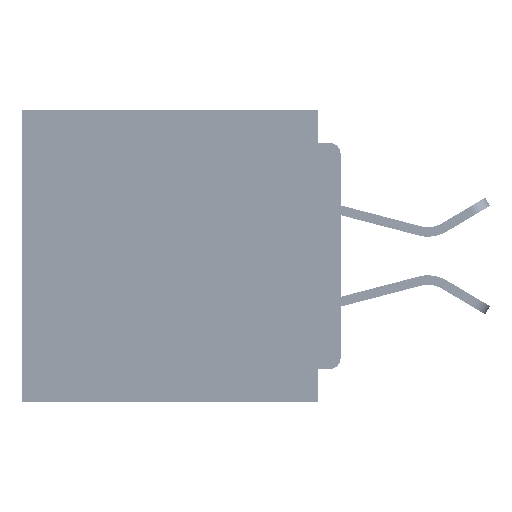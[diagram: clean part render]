
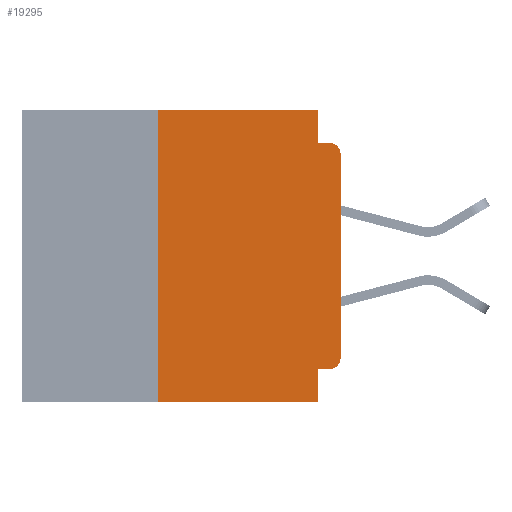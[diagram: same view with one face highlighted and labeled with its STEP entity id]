
A CAD part, left-side view. The second image highlights one B-rep face of the part: STEP entity #19295.
In plain terms, the highlighted planar face has unit normal (-1, 0, 0).
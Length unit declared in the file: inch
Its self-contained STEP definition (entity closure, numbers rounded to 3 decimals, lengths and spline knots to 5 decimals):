
#38 = PLANE ( 'NONE',  #16601 ) ;
#357 = CARTESIAN_POINT ( 'NONE',  ( 0., 0.25, -0.4 ) ) ;
#648 = DIRECTION ( 'NONE',  ( 0., 0., -1. ) ) ;
#830 = LINE ( 'NONE', #15773, #28668 ) ;
#1079 = VECTOR ( 'NONE', #26083, 39.37008 ) ;
#1973 = VERTEX_POINT ( 'NONE', #3109 ) ;
#2533 = CARTESIAN_POINT ( 'NONE',  ( 0., 0.031, -0.045 ) ) ;
#3109 = CARTESIAN_POINT ( 'NONE',  ( 0., 0.031, 0. ) ) ;
#3310 = EDGE_LOOP ( 'NONE', ( #9138, #9991, #10525, #57037, #30089, #4718, #67123, #20669, #21272, #42028 ) ) ;
#4119 = DIRECTION ( 'NONE',  ( 0., 0., -1. ) ) ;
#4718 = ORIENTED_EDGE ( 'NONE', *, *, #27947, .F. ) ;
#5754 = CARTESIAN_POINT ( 'NONE',  ( 0., 0.031, 0. ) ) ;
#7017 = CARTESIAN_POINT ( 'NONE',  ( 0., 0.015, -0.34 ) ) ;
#8883 = VECTOR ( 'NONE', #55466, 39.37008 ) ;
#9138 = ORIENTED_EDGE ( 'NONE', *, *, #44652, .T. ) ;
#9991 = ORIENTED_EDGE ( 'NONE', *, *, #26173, .T. ) ;
#10525 = ORIENTED_EDGE ( 'NONE', *, *, #39951, .F. ) ;
#12321 = DIRECTION ( 'NONE',  ( 0., 0., -1. ) ) ;
#14378 = VECTOR ( 'NONE', #648, 39.37008 ) ;
#15121 = LINE ( 'NONE', #20859, #1079 ) ;
#15773 = CARTESIAN_POINT ( 'NONE',  ( 0., 0., -0.045 ) ) ;
#16601 = AXIS2_PLACEMENT_3D ( 'NONE', #21153, #26368, #62753 ) ;
#16713 = VERTEX_POINT ( 'NONE', #2533 ) ;
#18641 = DIRECTION ( 'NONE',  ( 0., 0., 1. ) ) ;
#19295 = ADVANCED_FACE ( 'NONE', ( #60668 ), #38, .F. ) ;
#19976 = CARTESIAN_POINT ( 'NONE',  ( 0., 0.031, -0.4 ) ) ;
#20669 = ORIENTED_EDGE ( 'NONE', *, *, #38235, .F. ) ;
#20859 = CARTESIAN_POINT ( 'NONE',  ( 0., 0.031, -0.4 ) ) ;
#21153 = CARTESIAN_POINT ( 'NONE',  ( 0., 0.437, 0. ) ) ;
#21272 = ORIENTED_EDGE ( 'NONE', *, *, #29369, .F. ) ;
#21910 = VERTEX_POINT ( 'NONE', #357 ) ;
#24305 = VERTEX_POINT ( 'NONE', #26837 ) ;
#25367 = EDGE_CURVE ( 'NONE', #21910, #33306, #56587, .T. ) ;
#25763 = AXIS2_PLACEMENT_3D ( 'NONE', #7017, #43482, #12321 ) ;
#26083 = DIRECTION ( 'NONE',  ( 0., 0., -1. ) ) ;
#26173 = EDGE_CURVE ( 'NONE', #30161, #24305, #41852, .T. ) ;
#26368 = DIRECTION ( 'NONE',  ( 1., 0., 0. ) ) ;
#26810 = VERTEX_POINT ( 'NONE', #56219 ) ;
#26837 = CARTESIAN_POINT ( 'NONE',  ( 0., 0.015, -0.045 ) ) ;
#27947 = EDGE_CURVE ( 'NONE', #21910, #54724, #48153, .T. ) ;
#28179 = LINE ( 'NONE', #5754, #14378 ) ;
#28668 = VECTOR ( 'NONE', #52113, 39.37008 ) ;
#29369 = EDGE_CURVE ( 'NONE', #45812, #42485, #50404, .T. ) ;
#30089 = ORIENTED_EDGE ( 'NONE', *, *, #58222, .F. ) ;
#30161 = VERTEX_POINT ( 'NONE', #41069 ) ;
#31523 = DIRECTION ( 'NONE',  ( 0., -1., 0. ) ) ;
#33306 = VERTEX_POINT ( 'NONE', #19976 ) ;
#35358 = DIRECTION ( 'NONE',  ( -1., 0., 0. ) ) ;
#38235 = EDGE_CURVE ( 'NONE', #42485, #33306, #15121, .T. ) ;
#39951 = EDGE_CURVE ( 'NONE', #16713, #24305, #830, .T. ) ;
#40610 = AXIS2_PLACEMENT_3D ( 'NONE', #66527, #35358, #4119 ) ;
#41069 = CARTESIAN_POINT ( 'NONE',  ( 0., 0., -0.06 ) ) ;
#41627 = CARTESIAN_POINT ( 'NONE',  ( 0., 0.015, -0.355 ) ) ;
#41852 = CIRCLE ( 'NONE', #40610, 0.015 ) ;
#42028 = ORIENTED_EDGE ( 'NONE', *, *, #62318, .T. ) ;
#42031 = CARTESIAN_POINT ( 'NONE',  ( 0., 0.437, 0. ) ) ;
#42485 = VERTEX_POINT ( 'NONE', #56438 ) ;
#42767 = VECTOR ( 'NONE', #43662, 39.37008 ) ;
#43482 = DIRECTION ( 'NONE',  ( -1., 0., 0. ) ) ;
#43662 = DIRECTION ( 'NONE',  ( 0., -1., 0. ) ) ;
#44604 = LINE ( 'NONE', #42031, #58425 ) ;
#44652 = EDGE_CURVE ( 'NONE', #26810, #30161, #59941, .T. ) ;
#45812 = VERTEX_POINT ( 'NONE', #41627 ) ;
#47697 = VECTOR ( 'NONE', #18641, 39.37008 ) ;
#48153 = LINE ( 'NONE', #59299, #60395 ) ;
#49054 = DIRECTION ( 'NONE',  ( 0., 0., 1. ) ) ;
#50237 = CARTESIAN_POINT ( 'NONE',  ( 0., 0., -0.355 ) ) ;
#50404 = LINE ( 'NONE', #50237, #8883 ) ;
#52113 = DIRECTION ( 'NONE',  ( 0., -1., 0. ) ) ;
#54724 = VERTEX_POINT ( 'NONE', #59053 ) ;
#55005 = CARTESIAN_POINT ( 'NONE',  ( 0., 0., 0. ) ) ;
#55466 = DIRECTION ( 'NONE',  ( 0., 1., 0. ) ) ;
#56219 = CARTESIAN_POINT ( 'NONE',  ( 0., 0., -0.34 ) ) ;
#56438 = CARTESIAN_POINT ( 'NONE',  ( 0., 0.031, -0.355 ) ) ;
#56587 = LINE ( 'NONE', #59116, #42767 ) ;
#57037 = ORIENTED_EDGE ( 'NONE', *, *, #65211, .F. ) ;
#58222 = EDGE_CURVE ( 'NONE', #54724, #1973, #44604, .T. ) ;
#58425 = VECTOR ( 'NONE', #31523, 39.37008 ) ;
#59053 = CARTESIAN_POINT ( 'NONE',  ( 0., 0.25, 0. ) ) ;
#59116 = CARTESIAN_POINT ( 'NONE',  ( 0., 0.437, -0.4 ) ) ;
#59299 = CARTESIAN_POINT ( 'NONE',  ( 0., 0.25, -0.4 ) ) ;
#59941 = LINE ( 'NONE', #55005, #47697 ) ;
#60395 = VECTOR ( 'NONE', #49054, 39.37008 ) ;
#60668 = FACE_OUTER_BOUND ( 'NONE', #3310, .T. ) ;
#62318 = EDGE_CURVE ( 'NONE', #45812, #26810, #66872, .T. ) ;
#62753 = DIRECTION ( 'NONE',  ( 0., 0., -1. ) ) ;
#65211 = EDGE_CURVE ( 'NONE', #1973, #16713, #28179, .T. ) ;
#66527 = CARTESIAN_POINT ( 'NONE',  ( 0., 0.015, -0.06 ) ) ;
#66872 = CIRCLE ( 'NONE', #25763, 0.015 ) ;
#67123 = ORIENTED_EDGE ( 'NONE', *, *, #25367, .T. ) ;
